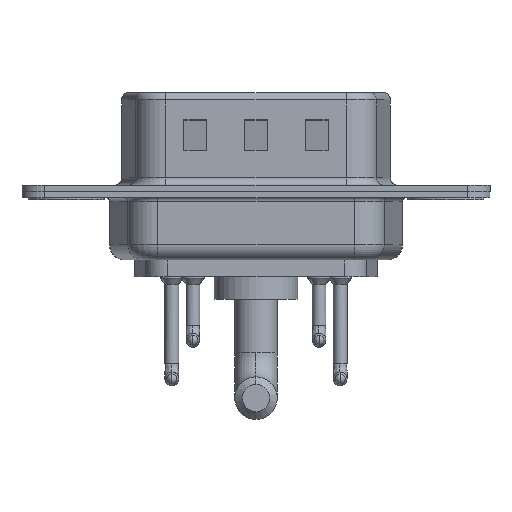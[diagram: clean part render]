
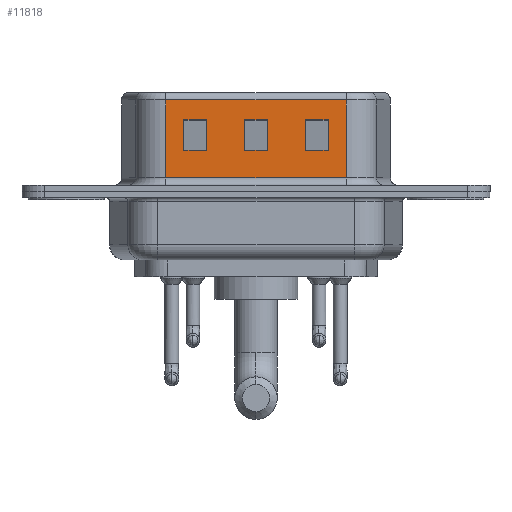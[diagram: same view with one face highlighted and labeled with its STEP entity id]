
A CAD part, front view. The second image highlights one B-rep face of the part: STEP entity #11818.
In plain terms, the highlighted planar face has unit normal (0, -1, 0).
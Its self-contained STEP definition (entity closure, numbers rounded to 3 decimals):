
#78 = CARTESIAN_POINT ( 'NONE',  ( 13.25, -4.55, 6.52 ) ) ;
#333 = LINE ( 'NONE', #13570, #5902 ) ;
#397 = VERTEX_POINT ( 'NONE', #8939 ) ;
#538 = EDGE_CURVE ( 'NONE', #10209, #7437, #15776, .T. ) ;
#541 = EDGE_CURVE ( 'NONE', #13912, #10209, #8048, .T. ) ;
#623 = VECTOR ( 'NONE', #15704, 1000. ) ;
#784 = FACE_BOUND ( 'NONE', #14277, .T. ) ;
#854 = VECTOR ( 'NONE', #3006, 1000. ) ;
#903 = CARTESIAN_POINT ( 'NONE',  ( 17.25, -4.55, 2.705 ) ) ;
#967 = PLANE ( 'NONE',  #2785 ) ;
#1001 = EDGE_CURVE ( 'NONE', #14620, #10258, #7852, .T. ) ;
#1042 = DIRECTION ( 'NONE',  ( -1., 0., 0. ) ) ;
#1089 = CARTESIAN_POINT ( 'NONE',  ( 6.549, -4.55, 6.02 ) ) ;
#1159 = CARTESIAN_POINT ( 'NONE',  ( 18.451, -4.55, 6.52 ) ) ;
#1296 = CARTESIAN_POINT ( 'NONE',  ( 17.25, -4.55, 4.705 ) ) ;
#1331 = DIRECTION ( 'NONE',  ( 0., 0., -1. ) ) ;
#1378 = VERTEX_POINT ( 'NONE', #4553 ) ;
#1640 = ORIENTED_EDGE ( 'NONE', *, *, #5547, .F. ) ;
#1788 = EDGE_CURVE ( 'NONE', #7305, #13912, #5854, .T. ) ;
#1873 = VECTOR ( 'NONE', #9029, 1000. ) ;
#2463 = VECTOR ( 'NONE', #15809, 1000. ) ;
#2467 = CARTESIAN_POINT ( 'NONE',  ( 18.451, -4.55, 6.02 ) ) ;
#2483 = EDGE_CURVE ( 'NONE', #10258, #1378, #5659, .T. ) ;
#2730 = EDGE_CURVE ( 'NONE', #5653, #10963, #7706, .T. ) ;
#2785 = AXIS2_PLACEMENT_3D ( 'NONE', #11614, #17022, #10275 ) ;
#3006 = DIRECTION ( 'NONE',  ( 0., 0., 1. ) ) ;
#3220 = ORIENTED_EDGE ( 'NONE', *, *, #538, .T. ) ;
#3252 = CARTESIAN_POINT ( 'NONE',  ( 11.75, -4.55, 4.705 ) ) ;
#3434 = ORIENTED_EDGE ( 'NONE', *, *, #5988, .T. ) ;
#3452 = FACE_BOUND ( 'NONE', #11742, .T. ) ;
#3548 = VERTEX_POINT ( 'NONE', #11898 ) ;
#3608 = CARTESIAN_POINT ( 'NONE',  ( 15.75, -4.55, 6.52 ) ) ;
#3728 = EDGE_LOOP ( 'NONE', ( #6083, #7156, #3220, #13336 ) ) ;
#3817 = VECTOR ( 'NONE', #11547, 1000. ) ;
#3823 = CARTESIAN_POINT ( 'NONE',  ( 18.451, -4.55, 4.705 ) ) ;
#4008 = LINE ( 'NONE', #3823, #2463 ) ;
#4149 = DIRECTION ( 'NONE',  ( 0., 0., -1. ) ) ;
#4300 = VECTOR ( 'NONE', #13942, 1000. ) ;
#4532 = EDGE_CURVE ( 'NONE', #10963, #16425, #14376, .T. ) ;
#4553 = CARTESIAN_POINT ( 'NONE',  ( 7.75, -4.55, 4.705 ) ) ;
#4682 = VERTEX_POINT ( 'NONE', #2467 ) ;
#4791 = LINE ( 'NONE', #1159, #15119 ) ;
#5227 = EDGE_CURVE ( 'NONE', #12443, #3548, #6697, .T. ) ;
#5547 = EDGE_CURVE ( 'NONE', #4682, #9775, #4791, .T. ) ;
#5653 = VERTEX_POINT ( 'NONE', #16067 ) ;
#5659 = LINE ( 'NONE', #11083, #854 ) ;
#5854 = LINE ( 'NONE', #11270, #17272 ) ;
#5902 = VECTOR ( 'NONE', #14901, 1000. ) ;
#5988 = EDGE_CURVE ( 'NONE', #11051, #5653, #14818, .T. ) ;
#6083 = ORIENTED_EDGE ( 'NONE', *, *, #1788, .T. ) ;
#6192 = FACE_OUTER_BOUND ( 'NONE', #10530, .T. ) ;
#6697 = LINE ( 'NONE', #12202, #12000 ) ;
#7156 = ORIENTED_EDGE ( 'NONE', *, *, #541, .T. ) ;
#7181 = EDGE_CURVE ( 'NONE', #7437, #7305, #17273, .T. ) ;
#7305 = VERTEX_POINT ( 'NONE', #1296 ) ;
#7437 = VERTEX_POINT ( 'NONE', #15734 ) ;
#7555 = CARTESIAN_POINT ( 'NONE',  ( 9.25, -4.55, 6.52 ) ) ;
#7706 = LINE ( 'NONE', #16924, #8232 ) ;
#7845 = CARTESIAN_POINT ( 'NONE',  ( 18.451, -4.55, 0.9 ) ) ;
#7852 = LINE ( 'NONE', #9364, #12418 ) ;
#7910 = CARTESIAN_POINT ( 'NONE',  ( 15.75, -4.55, 2.705 ) ) ;
#8048 = LINE ( 'NONE', #14628, #8677 ) ;
#8117 = DIRECTION ( 'NONE',  ( 0., 0., -1. ) ) ;
#8232 = VECTOR ( 'NONE', #1042, 1000. ) ;
#8329 = VECTOR ( 'NONE', #15956, 1000. ) ;
#8583 = EDGE_CURVE ( 'NONE', #4682, #12443, #13345, .T. ) ;
#8650 = ORIENTED_EDGE ( 'NONE', *, *, #8583, .T. ) ;
#8677 = VECTOR ( 'NONE', #11865, 1000. ) ;
#8683 = LINE ( 'NONE', #15094, #4300 ) ;
#8872 = FACE_BOUND ( 'NONE', #3728, .T. ) ;
#8939 = CARTESIAN_POINT ( 'NONE',  ( 9.25, -4.55, 4.705 ) ) ;
#9029 = DIRECTION ( 'NONE',  ( 0., 0., 1. ) ) ;
#9176 = CARTESIAN_POINT ( 'NONE',  ( 18.451, -4.55, 6.02 ) ) ;
#9364 = CARTESIAN_POINT ( 'NONE',  ( 14.451, -4.55, 2.705 ) ) ;
#9513 = ORIENTED_EDGE ( 'NONE', *, *, #2730, .T. ) ;
#9775 = VERTEX_POINT ( 'NONE', #7845 ) ;
#10117 = LINE ( 'NONE', #7555, #3817 ) ;
#10210 = EDGE_CURVE ( 'NONE', #16425, #11051, #4008, .T. ) ;
#10209 = VERTEX_POINT ( 'NONE', #7910 ) ;
#10258 = VERTEX_POINT ( 'NONE', #10655 ) ;
#10275 = DIRECTION ( 'NONE',  ( -1., 0., 0. ) ) ;
#10530 = EDGE_LOOP ( 'NONE', ( #1640, #8650, #11641, #11454 ) ) ;
#10616 = CARTESIAN_POINT ( 'NONE',  ( 22.451, -4.55, 4.705 ) ) ;
#10655 = CARTESIAN_POINT ( 'NONE',  ( 7.75, -4.55, 2.705 ) ) ;
#10963 = VERTEX_POINT ( 'NONE', #11678 ) ;
#11051 = VERTEX_POINT ( 'NONE', #12031 ) ;
#11083 = CARTESIAN_POINT ( 'NONE',  ( 7.75, -4.55, 6.52 ) ) ;
#11270 = CARTESIAN_POINT ( 'NONE',  ( 17.25, -4.55, 6.52 ) ) ;
#11454 = ORIENTED_EDGE ( 'NONE', *, *, #17069, .T. ) ;
#11472 = VECTOR ( 'NONE', #13171, 1000. ) ;
#11483 = ORIENTED_EDGE ( 'NONE', *, *, #4532, .T. ) ;
#11547 = DIRECTION ( 'NONE',  ( 0., 0., -1. ) ) ;
#11610 = CARTESIAN_POINT ( 'NONE',  ( 11.75, -4.55, 6.52 ) ) ;
#11614 = CARTESIAN_POINT ( 'NONE',  ( 18.451, -4.55, 6.52 ) ) ;
#11618 = ORIENTED_EDGE ( 'NONE', *, *, #1001, .T. ) ;
#11641 = ORIENTED_EDGE ( 'NONE', *, *, #5227, .T. ) ;
#11678 = CARTESIAN_POINT ( 'NONE',  ( 11.75, -4.55, 2.705 ) ) ;
#11742 = EDGE_LOOP ( 'NONE', ( #13271, #11618, #17431, #16323 ) ) ;
#11818 = ADVANCED_FACE ( 'NONE', ( #3452, #8872, #784, #6192 ), #967, .F. ) ;
#11865 = DIRECTION ( 'NONE',  ( -1., 0., 0. ) ) ;
#11898 = CARTESIAN_POINT ( 'NONE',  ( 6.549, -4.55, 0.9 ) ) ;
#12000 = VECTOR ( 'NONE', #8117, 1000. ) ;
#12003 = CARTESIAN_POINT ( 'NONE',  ( 9.25, -4.55, 2.705 ) ) ;
#12031 = CARTESIAN_POINT ( 'NONE',  ( 13.25, -4.55, 4.705 ) ) ;
#12202 = CARTESIAN_POINT ( 'NONE',  ( 6.549, -4.55, 6.52 ) ) ;
#12418 = VECTOR ( 'NONE', #13266, 1000. ) ;
#12443 = VERTEX_POINT ( 'NONE', #1089 ) ;
#13171 = DIRECTION ( 'NONE',  ( -1., 0., 0. ) ) ;
#13266 = DIRECTION ( 'NONE',  ( -1., 0., 0. ) ) ;
#13271 = ORIENTED_EDGE ( 'NONE', *, *, #13820, .T. ) ;
#13336 = ORIENTED_EDGE ( 'NONE', *, *, #7181, .T. ) ;
#13345 = LINE ( 'NONE', #9176, #11472 ) ;
#13352 = EDGE_CURVE ( 'NONE', #1378, #397, #333, .T. ) ;
#13570 = CARTESIAN_POINT ( 'NONE',  ( 14.451, -4.55, 4.705 ) ) ;
#13820 = EDGE_CURVE ( 'NONE', #397, #14620, #10117, .T. ) ;
#13912 = VERTEX_POINT ( 'NONE', #903 ) ;
#13942 = DIRECTION ( 'NONE',  ( 1., 0., 0. ) ) ;
#14277 = EDGE_LOOP ( 'NONE', ( #15148, #3434, #9513, #11483 ) ) ;
#14376 = LINE ( 'NONE', #11610, #623 ) ;
#14620 = VERTEX_POINT ( 'NONE', #12003 ) ;
#14628 = CARTESIAN_POINT ( 'NONE',  ( 22.451, -4.55, 2.705 ) ) ;
#14818 = LINE ( 'NONE', #78, #16812 ) ;
#14901 = DIRECTION ( 'NONE',  ( 1., 0., 0. ) ) ;
#15094 = CARTESIAN_POINT ( 'NONE',  ( 18.451, -4.55, 0.9 ) ) ;
#15119 = VECTOR ( 'NONE', #1331, 1000. ) ;
#15148 = ORIENTED_EDGE ( 'NONE', *, *, #10210, .T. ) ;
#15704 = DIRECTION ( 'NONE',  ( 0., 0., 1. ) ) ;
#15734 = CARTESIAN_POINT ( 'NONE',  ( 15.75, -4.55, 4.705 ) ) ;
#15776 = LINE ( 'NONE', #3608, #1873 ) ;
#15809 = DIRECTION ( 'NONE',  ( 1., 0., 0. ) ) ;
#15956 = DIRECTION ( 'NONE',  ( 1., 0., 0. ) ) ;
#16067 = CARTESIAN_POINT ( 'NONE',  ( 13.25, -4.55, 2.705 ) ) ;
#16323 = ORIENTED_EDGE ( 'NONE', *, *, #13352, .T. ) ;
#16425 = VERTEX_POINT ( 'NONE', #3252 ) ;
#16685 = DIRECTION ( 'NONE',  ( 0., 0., -1. ) ) ;
#16812 = VECTOR ( 'NONE', #4149, 1000. ) ;
#16924 = CARTESIAN_POINT ( 'NONE',  ( 18.451, -4.55, 2.705 ) ) ;
#17022 = DIRECTION ( 'NONE',  ( 0., 1., 0. ) ) ;
#17069 = EDGE_CURVE ( 'NONE', #3548, #9775, #8683, .T. ) ;
#17272 = VECTOR ( 'NONE', #16685, 1000. ) ;
#17273 = LINE ( 'NONE', #10616, #8329 ) ;
#17431 = ORIENTED_EDGE ( 'NONE', *, *, #2483, .T. ) ;
